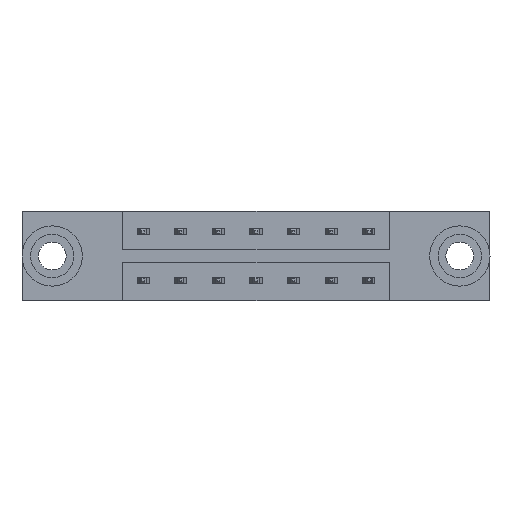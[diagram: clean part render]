
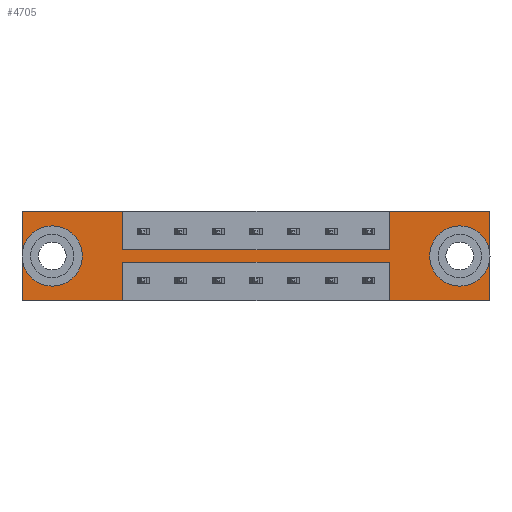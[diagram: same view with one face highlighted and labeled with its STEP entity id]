
A CAD part, front view. The second image highlights one B-rep face of the part: STEP entity #4705.
In plain terms, the highlighted planar face has unit normal (0, -1, 0).
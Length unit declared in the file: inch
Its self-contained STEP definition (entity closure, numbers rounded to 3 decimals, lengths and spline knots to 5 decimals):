
#63 = LINE ( 'NONE', #9096, #7668 ) ;
#65 = VERTEX_POINT ( 'NONE', #6486 ) ;
#73 = ORIENTED_EDGE ( 'NONE', *, *, #7984, .F. ) ;
#80 = VERTEX_POINT ( 'NONE', #6528 ) ;
#106 = FACE_BOUND ( 'NONE', #7386, .T. ) ;
#301 = CARTESIAN_POINT ( 'NONE',  ( 1.94, 0., -0.37 ) ) ;
#315 = CARTESIAN_POINT ( 'NONE',  ( 0.4175, 0., -0.1585 ) ) ;
#340 = ORIENTED_EDGE ( 'NONE', *, *, #725, .F. ) ;
#442 = ORIENTED_EDGE ( 'NONE', *, *, #5778, .T. ) ;
#459 = EDGE_CURVE ( 'NONE', #988, #1750, #8556, .T. ) ;
#725 = EDGE_CURVE ( 'NONE', #80, #3107, #8185, .T. ) ;
#787 = CARTESIAN_POINT ( 'NONE',  ( 0.125, 0., -0.107 ) ) ;
#792 = DIRECTION ( 'NONE',  ( 0., 0., 1. ) ) ;
#794 = DIRECTION ( 'NONE',  ( 0., -1., 0. ) ) ;
#827 = CARTESIAN_POINT ( 'NONE',  ( 0.125, 0., -0.185 ) ) ;
#857 = LINE ( 'NONE', #4710, #7708 ) ;
#888 = CIRCLE ( 'NONE', #2931, 0.078 ) ;
#969 = EDGE_CURVE ( 'NONE', #4592, #80, #5034, .T. ) ;
#988 = VERTEX_POINT ( 'NONE', #1267 ) ;
#1108 = CARTESIAN_POINT ( 'NONE',  ( 0.4175, 0., -0.37 ) ) ;
#1123 = LINE ( 'NONE', #3399, #5571 ) ;
#1218 = CARTESIAN_POINT ( 'NONE',  ( 0.4175, 0., -0.2115 ) ) ;
#1239 = VERTEX_POINT ( 'NONE', #787 ) ;
#1267 = CARTESIAN_POINT ( 'NONE',  ( 1.815, 0., -0.263 ) ) ;
#1293 = LINE ( 'NONE', #6621, #9533 ) ;
#1422 = CARTESIAN_POINT ( 'NONE',  ( 1.5225, 0., -0.1585 ) ) ;
#1560 = CARTESIAN_POINT ( 'NONE',  ( 0., 0., 0. ) ) ;
#1586 = VECTOR ( 'NONE', #6948, 39.37008 ) ;
#1655 = LINE ( 'NONE', #7660, #3339 ) ;
#1668 = ORIENTED_EDGE ( 'NONE', *, *, #459, .T. ) ;
#1750 = VERTEX_POINT ( 'NONE', #6967 ) ;
#1787 = EDGE_CURVE ( 'NONE', #1239, #5360, #888, .T. ) ;
#1814 = CARTESIAN_POINT ( 'NONE',  ( 0.4175, 0., 0. ) ) ;
#1821 = CARTESIAN_POINT ( 'NONE',  ( 0., 0., -0.37 ) ) ;
#1849 = AXIS2_PLACEMENT_3D ( 'NONE', #7529, #794, #8172 ) ;
#1891 = EDGE_CURVE ( 'NONE', #2841, #4836, #1293, .T. ) ;
#2196 = CARTESIAN_POINT ( 'NONE',  ( 1.5225, 0., -0.37 ) ) ;
#2338 = DIRECTION ( 'NONE',  ( 0., 1., 0. ) ) ;
#2363 = DIRECTION ( 'NONE',  ( 0., 0., 1. ) ) ;
#2422 = ORIENTED_EDGE ( 'NONE', *, *, #2467, .F. ) ;
#2467 = EDGE_CURVE ( 'NONE', #5742, #3589, #8570, .T. ) ;
#2506 = CIRCLE ( 'NONE', #3761, 0.078 ) ;
#2517 = DIRECTION ( 'NONE',  ( 0., 0., -1. ) ) ;
#2666 = LINE ( 'NONE', #315, #9259 ) ;
#2841 = VERTEX_POINT ( 'NONE', #1560 ) ;
#2867 = EDGE_CURVE ( 'NONE', #5360, #1239, #4505, .T. ) ;
#2896 = DIRECTION ( 'NONE',  ( 0., 0., 1. ) ) ;
#2931 = AXIS2_PLACEMENT_3D ( 'NONE', #8590, #7701, #3973 ) ;
#2997 = ORIENTED_EDGE ( 'NONE', *, *, #969, .F. ) ;
#3083 = EDGE_LOOP ( 'NONE', ( #4182, #5294 ) ) ;
#3107 = VERTEX_POINT ( 'NONE', #1108 ) ;
#3138 = CARTESIAN_POINT ( 'NONE',  ( 1.815, 0., -0.185 ) ) ;
#3213 = EDGE_LOOP ( 'NONE', ( #4249, #4457, #2422, #9048, #73, #7587, #4504, #7918, #7290, #8283, #340, #2997 ) ) ;
#3339 = VECTOR ( 'NONE', #6976, 39.37008 ) ;
#3399 = CARTESIAN_POINT ( 'NONE',  ( 0., 0., -0.37 ) ) ;
#3422 = CARTESIAN_POINT ( 'NONE',  ( 1.815, 0., -0.185 ) ) ;
#3589 = VERTEX_POINT ( 'NONE', #301 ) ;
#3759 = DIRECTION ( 'NONE',  ( 0., 0., -1. ) ) ;
#3761 = AXIS2_PLACEMENT_3D ( 'NONE', #3138, #2338, #6234 ) ;
#3782 = EDGE_CURVE ( 'NONE', #3107, #5035, #1123, .T. ) ;
#3833 = DIRECTION ( 'NONE',  ( 0., 0., 1. ) ) ;
#3872 = EDGE_CURVE ( 'NONE', #5035, #2841, #5960, .T. ) ;
#3876 = VERTEX_POINT ( 'NONE', #2196 ) ;
#3973 = DIRECTION ( 'NONE',  ( 0., 0., 1. ) ) ;
#4118 = VECTOR ( 'NONE', #792, 39.37008 ) ;
#4182 = ORIENTED_EDGE ( 'NONE', *, *, #1787, .T. ) ;
#4249 = ORIENTED_EDGE ( 'NONE', *, *, #4766, .F. ) ;
#4318 = AXIS2_PLACEMENT_3D ( 'NONE', #3422, #9362, #7147 ) ;
#4444 = FACE_BOUND ( 'NONE', #3083, .T. ) ;
#4457 = ORIENTED_EDGE ( 'NONE', *, *, #7621, .F. ) ;
#4482 = CARTESIAN_POINT ( 'NONE',  ( 0., 0., 0. ) ) ;
#4504 = ORIENTED_EDGE ( 'NONE', *, *, #7513, .F. ) ;
#4505 = CIRCLE ( 'NONE', #5764, 0.078 ) ;
#4545 = FACE_OUTER_BOUND ( 'NONE', #3213, .T. ) ;
#4592 = VERTEX_POINT ( 'NONE', #8583 ) ;
#4705 = ADVANCED_FACE ( 'NONE', ( #106, #4444, #4545 ), #8371, .T. ) ;
#4710 = CARTESIAN_POINT ( 'NONE',  ( 0.4175, 0., -0.1585 ) ) ;
#4766 = EDGE_CURVE ( 'NONE', #3876, #4592, #63, .T. ) ;
#4819 = CARTESIAN_POINT ( 'NONE',  ( 1.94, 0., 0. ) ) ;
#4836 = VERTEX_POINT ( 'NONE', #1814 ) ;
#4941 = VECTOR ( 'NONE', #8747, 39.37008 ) ;
#5034 = LINE ( 'NONE', #1218, #4941 ) ;
#5035 = VERTEX_POINT ( 'NONE', #5727 ) ;
#5294 = ORIENTED_EDGE ( 'NONE', *, *, #2867, .T. ) ;
#5360 = VERTEX_POINT ( 'NONE', #5522 ) ;
#5375 = DIRECTION ( 'NONE',  ( 0., 1., 0. ) ) ;
#5459 = CARTESIAN_POINT ( 'NONE',  ( 1.5225, 0., -0.1585 ) ) ;
#5522 = CARTESIAN_POINT ( 'NONE',  ( 0.125, 0., -0.263 ) ) ;
#5571 = VECTOR ( 'NONE', #7165, 39.37008 ) ;
#5727 = CARTESIAN_POINT ( 'NONE',  ( 0., 0., -0.37 ) ) ;
#5731 = VERTEX_POINT ( 'NONE', #5459 ) ;
#5742 = VERTEX_POINT ( 'NONE', #4819 ) ;
#5743 = VECTOR ( 'NONE', #3759, 39.37008 ) ;
#5764 = AXIS2_PLACEMENT_3D ( 'NONE', #827, #5375, #3833 ) ;
#5778 = EDGE_CURVE ( 'NONE', #1750, #988, #2506, .T. ) ;
#5789 = VECTOR ( 'NONE', #2896, 39.37008 ) ;
#5846 = DIRECTION ( 'NONE',  ( 1., 0., 0. ) ) ;
#5960 = LINE ( 'NONE', #4482, #5789 ) ;
#6234 = DIRECTION ( 'NONE',  ( 0., 0., -1. ) ) ;
#6374 = EDGE_CURVE ( 'NONE', #7191, #5731, #2666, .T. ) ;
#6486 = CARTESIAN_POINT ( 'NONE',  ( 1.5225, 0., 0. ) ) ;
#6509 = DIRECTION ( 'NONE',  ( 1., 0., 0. ) ) ;
#6528 = CARTESIAN_POINT ( 'NONE',  ( 0.4175, 0., -0.2115 ) ) ;
#6621 = CARTESIAN_POINT ( 'NONE',  ( 0., 0., 0. ) ) ;
#6948 = DIRECTION ( 'NONE',  ( -1., 0., 0. ) ) ;
#6967 = CARTESIAN_POINT ( 'NONE',  ( 1.815, 0., -0.107 ) ) ;
#6976 = DIRECTION ( 'NONE',  ( 1., 0., 0. ) ) ;
#7059 = CARTESIAN_POINT ( 'NONE',  ( 0.4175, 0., -0.1585 ) ) ;
#7147 = DIRECTION ( 'NONE',  ( 0., 0., -1. ) ) ;
#7165 = DIRECTION ( 'NONE',  ( -1., 0., 0. ) ) ;
#7191 = VERTEX_POINT ( 'NONE', #7059 ) ;
#7290 = ORIENTED_EDGE ( 'NONE', *, *, #3872, .F. ) ;
#7386 = EDGE_LOOP ( 'NONE', ( #442, #1668 ) ) ;
#7513 = EDGE_CURVE ( 'NONE', #4836, #7191, #857, .T. ) ;
#7529 = CARTESIAN_POINT ( 'NONE',  ( 0., 0., -0.37 ) ) ;
#7587 = ORIENTED_EDGE ( 'NONE', *, *, #6374, .F. ) ;
#7621 = EDGE_CURVE ( 'NONE', #3589, #3876, #8483, .T. ) ;
#7652 = VECTOR ( 'NONE', #2517, 39.37008 ) ;
#7660 = CARTESIAN_POINT ( 'NONE',  ( 0., 0., 0. ) ) ;
#7668 = VECTOR ( 'NONE', #2363, 39.37008 ) ;
#7689 = DIRECTION ( 'NONE',  ( 0., 0., -1. ) ) ;
#7701 = DIRECTION ( 'NONE',  ( 0., 1., 0. ) ) ;
#7708 = VECTOR ( 'NONE', #7689, 39.37008 ) ;
#7918 = ORIENTED_EDGE ( 'NONE', *, *, #1891, .F. ) ;
#7984 = EDGE_CURVE ( 'NONE', #5731, #65, #9694, .T. ) ;
#8132 = CARTESIAN_POINT ( 'NONE',  ( 0.4175, 0., -0.2115 ) ) ;
#8172 = DIRECTION ( 'NONE',  ( 0., 0., -1. ) ) ;
#8185 = LINE ( 'NONE', #8132, #5743 ) ;
#8283 = ORIENTED_EDGE ( 'NONE', *, *, #3782, .F. ) ;
#8371 = PLANE ( 'NONE',  #1849 ) ;
#8483 = LINE ( 'NONE', #1821, #1586 ) ;
#8525 = CARTESIAN_POINT ( 'NONE',  ( 1.94, 0., 0. ) ) ;
#8556 = CIRCLE ( 'NONE', #4318, 0.078 ) ;
#8570 = LINE ( 'NONE', #8525, #7652 ) ;
#8583 = CARTESIAN_POINT ( 'NONE',  ( 1.5225, 0., -0.2115 ) ) ;
#8590 = CARTESIAN_POINT ( 'NONE',  ( 0.125, 0., -0.185 ) ) ;
#8596 = EDGE_CURVE ( 'NONE', #65, #5742, #1655, .T. ) ;
#8747 = DIRECTION ( 'NONE',  ( -1., 0., 0. ) ) ;
#9048 = ORIENTED_EDGE ( 'NONE', *, *, #8596, .F. ) ;
#9096 = CARTESIAN_POINT ( 'NONE',  ( 1.5225, 0., -0.2115 ) ) ;
#9259 = VECTOR ( 'NONE', #6509, 39.37008 ) ;
#9362 = DIRECTION ( 'NONE',  ( 0., 1., 0. ) ) ;
#9533 = VECTOR ( 'NONE', #5846, 39.37008 ) ;
#9694 = LINE ( 'NONE', #1422, #4118 ) ;
